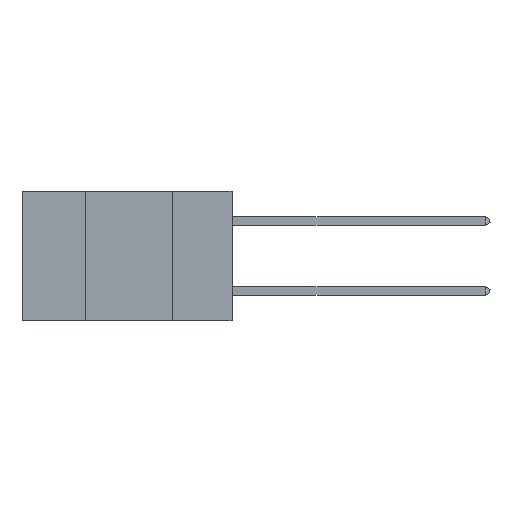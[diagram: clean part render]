
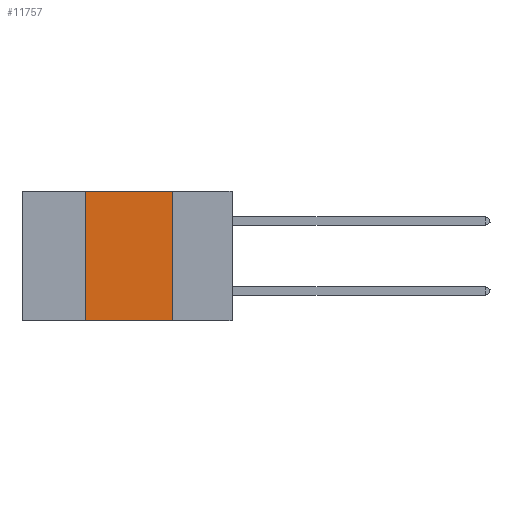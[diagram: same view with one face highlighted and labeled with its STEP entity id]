
A CAD part, left-side view. The second image highlights one B-rep face of the part: STEP entity #11757.
In plain terms, the highlighted planar face has unit normal (-1, 0, 0).
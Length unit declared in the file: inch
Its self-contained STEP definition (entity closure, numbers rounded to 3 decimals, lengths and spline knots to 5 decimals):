
#143 = VECTOR ( 'NONE', #12351, 39.37008 ) ;
#186 = AXIS2_PLACEMENT_3D ( 'NONE', #11512, #18991, #11347 ) ;
#1631 = DIRECTION ( 'NONE',  ( 0., 0., -1. ) ) ;
#3769 = VERTEX_POINT ( 'NONE', #7977 ) ;
#4546 = CARTESIAN_POINT ( 'NONE',  ( 0., 0.6, 0. ) ) ;
#4591 = LINE ( 'NONE', #14631, #143 ) ;
#6417 = CARTESIAN_POINT ( 'NONE',  ( 0., 0.17, 0. ) ) ;
#7222 = CARTESIAN_POINT ( 'NONE',  ( 0., 0.17, 0. ) ) ;
#7977 = CARTESIAN_POINT ( 'NONE',  ( 0., 0.42, 0. ) ) ;
#8132 = CARTESIAN_POINT ( 'NONE',  ( 0., 0.42, -0.37 ) ) ;
#8325 = LINE ( 'NONE', #6417, #15348 ) ;
#8329 = PLANE ( 'NONE',  #186 ) ;
#8656 = VERTEX_POINT ( 'NONE', #8132 ) ;
#9143 = EDGE_LOOP ( 'NONE', ( #28100, #11701, #17511, #21426 ) ) ;
#10512 = VECTOR ( 'NONE', #11261, 39.37008 ) ;
#11261 = DIRECTION ( 'NONE',  ( 0., -1., 0. ) ) ;
#11347 = DIRECTION ( 'NONE',  ( 0., 0., -1. ) ) ;
#11512 = CARTESIAN_POINT ( 'NONE',  ( 0., 0.6, 0. ) ) ;
#11701 = ORIENTED_EDGE ( 'NONE', *, *, #25717, .F. ) ;
#11757 = ADVANCED_FACE ( 'NONE', ( #27880 ), #8329, .F. ) ;
#12351 = DIRECTION ( 'NONE',  ( 0., 0., 1. ) ) ;
#14631 = CARTESIAN_POINT ( 'NONE',  ( 0., 0.42, 0. ) ) ;
#14983 = EDGE_CURVE ( 'NONE', #8656, #30329, #25455, .T. ) ;
#15348 = VECTOR ( 'NONE', #1631, 39.37008 ) ;
#15695 = LINE ( 'NONE', #4546, #10512 ) ;
#17511 = ORIENTED_EDGE ( 'NONE', *, *, #19337, .F. ) ;
#17877 = CARTESIAN_POINT ( 'NONE',  ( 0., 0.17, -0.37 ) ) ;
#18991 = DIRECTION ( 'NONE',  ( 1., 0., 0. ) ) ;
#19068 = EDGE_CURVE ( 'NONE', #26394, #30329, #8325, .T. ) ;
#19337 = EDGE_CURVE ( 'NONE', #8656, #3769, #4591, .T. ) ;
#21029 = VECTOR ( 'NONE', #25237, 39.37008 ) ;
#21426 = ORIENTED_EDGE ( 'NONE', *, *, #14983, .T. ) ;
#25237 = DIRECTION ( 'NONE',  ( 0., -1., 0. ) ) ;
#25455 = LINE ( 'NONE', #25532, #21029 ) ;
#25532 = CARTESIAN_POINT ( 'NONE',  ( 0., 0.6, -0.37 ) ) ;
#25717 = EDGE_CURVE ( 'NONE', #3769, #26394, #15695, .T. ) ;
#26394 = VERTEX_POINT ( 'NONE', #7222 ) ;
#27880 = FACE_OUTER_BOUND ( 'NONE', #9143, .T. ) ;
#28100 = ORIENTED_EDGE ( 'NONE', *, *, #19068, .F. ) ;
#30329 = VERTEX_POINT ( 'NONE', #17877 ) ;
